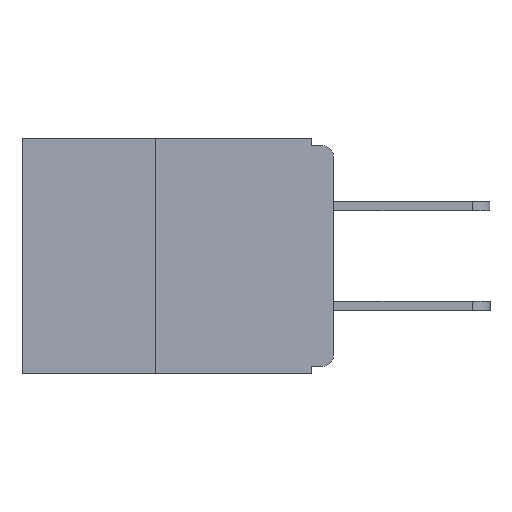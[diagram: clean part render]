
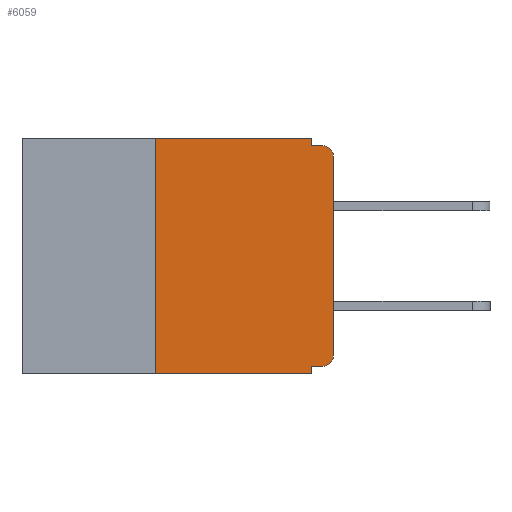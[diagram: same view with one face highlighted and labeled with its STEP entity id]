
A CAD part, left-side view. The second image highlights one B-rep face of the part: STEP entity #6059.
In plain terms, the highlighted planar face has unit normal (-1, 0, 0).
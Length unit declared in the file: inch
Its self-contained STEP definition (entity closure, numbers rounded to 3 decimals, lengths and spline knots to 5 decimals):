
#3 = EDGE_CURVE ( 'NONE', #1384, #10310, #2231, .T. ) ;
#67 = EDGE_CURVE ( 'NONE', #8518, #10468, #11204, .T. ) ;
#153 = CARTESIAN_POINT ( 'NONE',  ( 0., 0., 0. ) ) ;
#159 = DIRECTION ( 'NONE',  ( 0., 0., -1. ) ) ;
#511 = ORIENTED_EDGE ( 'NONE', *, *, #67, .T. ) ;
#735 = ORIENTED_EDGE ( 'NONE', *, *, #4891, .F. ) ;
#867 = CARTESIAN_POINT ( 'NONE',  ( 0., 0.437, 0. ) ) ;
#901 = VECTOR ( 'NONE', #1318, 39.37008 ) ;
#919 = CARTESIAN_POINT ( 'NONE',  ( 0., 0.25, -0.33 ) ) ;
#950 = ORIENTED_EDGE ( 'NONE', *, *, #2135, .T. ) ;
#1060 = CARTESIAN_POINT ( 'NONE',  ( 0., 0.25, -0.33 ) ) ;
#1261 = EDGE_CURVE ( 'NONE', #6061, #11201, #1648, .T. ) ;
#1280 = EDGE_CURVE ( 'NONE', #11201, #10002, #6182, .T. ) ;
#1318 = DIRECTION ( 'NONE',  ( 0., -1., 0. ) ) ;
#1384 = VERTEX_POINT ( 'NONE', #2478 ) ;
#1563 = DIRECTION ( 'NONE',  ( 0., 1., 0. ) ) ;
#1648 = LINE ( 'NONE', #11037, #9090 ) ;
#1698 = CARTESIAN_POINT ( 'NONE',  ( 0., 0.25, 0. ) ) ;
#2045 = CIRCLE ( 'NONE', #10149, 0.015 ) ;
#2135 = EDGE_CURVE ( 'NONE', #6139, #6123, #2045, .T. ) ;
#2231 = CIRCLE ( 'NONE', #10853, 0.015 ) ;
#2478 = CARTESIAN_POINT ( 'NONE',  ( 0., 0., -0.025 ) ) ;
#2499 = VECTOR ( 'NONE', #5720, 39.37008 ) ;
#2609 = PLANE ( 'NONE',  #3416 ) ;
#2671 = DIRECTION ( 'NONE',  ( 1., 0., 0. ) ) ;
#3148 = DIRECTION ( 'NONE',  ( 0., 0., -1. ) ) ;
#3406 = ORIENTED_EDGE ( 'NONE', *, *, #4173, .F. ) ;
#3416 = AXIS2_PLACEMENT_3D ( 'NONE', #867, #2671, #4342 ) ;
#3615 = VECTOR ( 'NONE', #4451, 39.37008 ) ;
#3623 = CARTESIAN_POINT ( 'NONE',  ( 0., 0.015, -0.32 ) ) ;
#3838 = ORIENTED_EDGE ( 'NONE', *, *, #1280, .F. ) ;
#3888 = CARTESIAN_POINT ( 'NONE',  ( 0., 0.437, -0.33 ) ) ;
#4012 = VECTOR ( 'NONE', #9980, 39.37008 ) ;
#4171 = CARTESIAN_POINT ( 'NONE',  ( 0., 0., -0.32 ) ) ;
#4173 = EDGE_CURVE ( 'NONE', #8518, #6061, #7325, .T. ) ;
#4221 = EDGE_LOOP ( 'NONE', ( #6737, #7368, #5557, #3838, #6053, #3406, #511, #5147, #735, #950 ) ) ;
#4276 = EDGE_CURVE ( 'NONE', #10002, #10310, #6932, .T. ) ;
#4342 = DIRECTION ( 'NONE',  ( 0., 0., -1. ) ) ;
#4451 = DIRECTION ( 'NONE',  ( 0., 0., 1. ) ) ;
#4469 = DIRECTION ( 'NONE',  ( 0., 0., -1. ) ) ;
#4891 = EDGE_CURVE ( 'NONE', #6139, #8574, #7447, .T. ) ;
#4902 = CARTESIAN_POINT ( 'NONE',  ( 0., 0.031, -0.33 ) ) ;
#4930 = DIRECTION ( 'NONE',  ( 0., -1., 0. ) ) ;
#5042 = CARTESIAN_POINT ( 'NONE',  ( 0., 0., -0.01 ) ) ;
#5147 = ORIENTED_EDGE ( 'NONE', *, *, #5825, .F. ) ;
#5154 = EDGE_CURVE ( 'NONE', #6123, #1384, #10658, .T. ) ;
#5341 = CARTESIAN_POINT ( 'NONE',  ( 0., 0.015, -0.01 ) ) ;
#5428 = CARTESIAN_POINT ( 'NONE',  ( 0., 0.015, -0.305 ) ) ;
#5557 = ORIENTED_EDGE ( 'NONE', *, *, #4276, .F. ) ;
#5720 = DIRECTION ( 'NONE',  ( 0., 0., -1. ) ) ;
#5825 = EDGE_CURVE ( 'NONE', #8574, #10468, #9796, .T. ) ;
#6053 = ORIENTED_EDGE ( 'NONE', *, *, #1261, .F. ) ;
#6059 = ADVANCED_FACE ( 'NONE', ( #10906 ), #2609, .F. ) ;
#6061 = VERTEX_POINT ( 'NONE', #1698 ) ;
#6123 = VERTEX_POINT ( 'NONE', #6249 ) ;
#6139 = VERTEX_POINT ( 'NONE', #3623 ) ;
#6182 = LINE ( 'NONE', #8323, #11018 ) ;
#6249 = CARTESIAN_POINT ( 'NONE',  ( 0., 0., -0.305 ) ) ;
#6737 = ORIENTED_EDGE ( 'NONE', *, *, #5154, .T. ) ;
#6932 = LINE ( 'NONE', #5042, #901 ) ;
#7046 = CARTESIAN_POINT ( 'NONE',  ( 0., 0.031, -0.32 ) ) ;
#7222 = CARTESIAN_POINT ( 'NONE',  ( 0., 0.015, -0.025 ) ) ;
#7325 = LINE ( 'NONE', #919, #3615 ) ;
#7368 = ORIENTED_EDGE ( 'NONE', *, *, #3, .T. ) ;
#7447 = LINE ( 'NONE', #4171, #11221 ) ;
#7874 = DIRECTION ( 'NONE',  ( 0., 0., 1. ) ) ;
#8022 = CARTESIAN_POINT ( 'NONE',  ( 0., 0.031, -0.01 ) ) ;
#8046 = DIRECTION ( 'NONE',  ( -1., 0., 0. ) ) ;
#8323 = CARTESIAN_POINT ( 'NONE',  ( 0., 0.031, 0. ) ) ;
#8518 = VERTEX_POINT ( 'NONE', #1060 ) ;
#8574 = VERTEX_POINT ( 'NONE', #7046 ) ;
#8614 = CARTESIAN_POINT ( 'NONE',  ( 0., 0.031, 0. ) ) ;
#9090 = VECTOR ( 'NONE', #4930, 39.37008 ) ;
#9796 = LINE ( 'NONE', #10123, #2499 ) ;
#9980 = DIRECTION ( 'NONE',  ( 0., -1., 0. ) ) ;
#10002 = VERTEX_POINT ( 'NONE', #8022 ) ;
#10123 = CARTESIAN_POINT ( 'NONE',  ( 0., 0.031, -0.33 ) ) ;
#10149 = AXIS2_PLACEMENT_3D ( 'NONE', #5428, #8046, #4469 ) ;
#10310 = VERTEX_POINT ( 'NONE', #5341 ) ;
#10468 = VERTEX_POINT ( 'NONE', #4902 ) ;
#10658 = LINE ( 'NONE', #153, #10928 ) ;
#10689 = DIRECTION ( 'NONE',  ( -1., 0., 0. ) ) ;
#10853 = AXIS2_PLACEMENT_3D ( 'NONE', #7222, #10689, #159 ) ;
#10906 = FACE_OUTER_BOUND ( 'NONE', #4221, .T. ) ;
#10928 = VECTOR ( 'NONE', #7874, 39.37008 ) ;
#11018 = VECTOR ( 'NONE', #3148, 39.37008 ) ;
#11037 = CARTESIAN_POINT ( 'NONE',  ( 0., 0.437, 0. ) ) ;
#11201 = VERTEX_POINT ( 'NONE', #8614 ) ;
#11204 = LINE ( 'NONE', #3888, #4012 ) ;
#11221 = VECTOR ( 'NONE', #1563, 39.37008 ) ;
